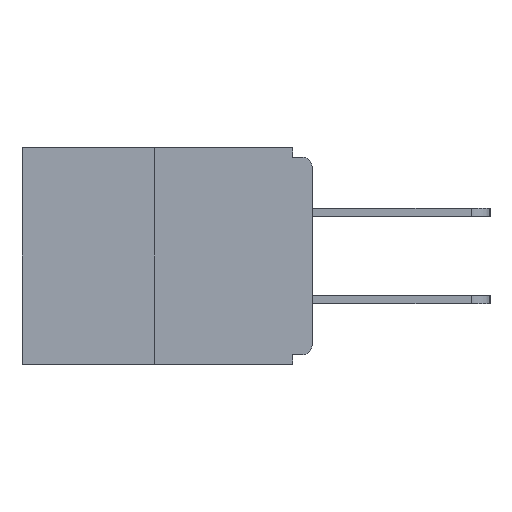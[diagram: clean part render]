
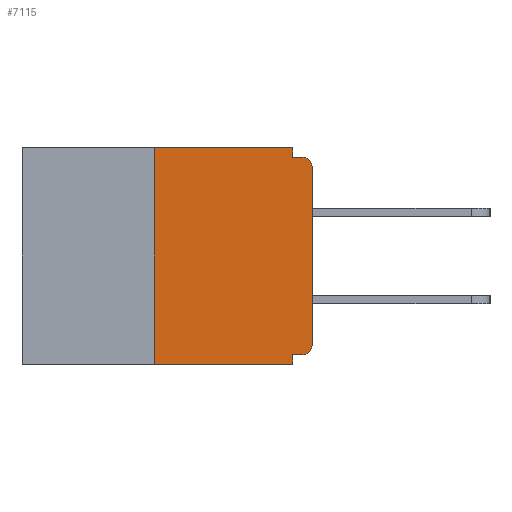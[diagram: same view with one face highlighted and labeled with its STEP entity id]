
A CAD part, left-side view. The second image highlights one B-rep face of the part: STEP entity #7115.
In plain terms, the highlighted planar face has unit normal (-1, 0, 0).
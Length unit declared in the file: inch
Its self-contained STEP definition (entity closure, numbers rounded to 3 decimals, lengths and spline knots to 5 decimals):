
#530 = AXIS2_PLACEMENT_3D ( 'NONE', #10379, #1969, #13027 ) ;
#532 = DIRECTION ( 'NONE',  ( 0., 0., -1. ) ) ;
#1036 = VECTOR ( 'NONE', #11976, 39.37008 ) ;
#1302 = VERTEX_POINT ( 'NONE', #10749 ) ;
#1969 = DIRECTION ( 'NONE',  ( -1., 0., 0. ) ) ;
#2118 = DIRECTION ( 'NONE',  ( 0., 0., -1. ) ) ;
#2387 = VERTEX_POINT ( 'NONE', #3374 ) ;
#2588 = EDGE_CURVE ( 'NONE', #21334, #2387, #24659, .T. ) ;
#2692 = LINE ( 'NONE', #12951, #17182 ) ;
#2912 = VECTOR ( 'NONE', #4541, 39.37008 ) ;
#3039 = ORIENTED_EDGE ( 'NONE', *, *, #25004, .F. ) ;
#3374 = CARTESIAN_POINT ( 'NONE',  ( 0., 0., -0.313 ) ) ;
#3795 = LINE ( 'NONE', #12334, #17183 ) ;
#4541 = DIRECTION ( 'NONE',  ( 0., -1., 0. ) ) ;
#4907 = CARTESIAN_POINT ( 'NONE',  ( 0., 0.46, 0. ) ) ;
#5122 = CARTESIAN_POINT ( 'NONE',  ( 0., 0.25, 0. ) ) ;
#5744 = EDGE_CURVE ( 'NONE', #2387, #20302, #27054, .T. ) ;
#6652 = LINE ( 'NONE', #24101, #2912 ) ;
#6734 = EDGE_LOOP ( 'NONE', ( #27359, #13438, #10868, #3039, #10901, #21600, #6792, #21544, #21994, #18970 ) ) ;
#6792 = ORIENTED_EDGE ( 'NONE', *, *, #5744, .T. ) ;
#7115 = ADVANCED_FACE ( 'NONE', ( #13035 ), #15799, .F. ) ;
#8331 = CARTESIAN_POINT ( 'NONE',  ( 0., 0.015, -0.015 ) ) ;
#9559 = DIRECTION ( 'NONE',  ( 0., 0., -1. ) ) ;
#9563 = EDGE_CURVE ( 'NONE', #1302, #16750, #18788, .T. ) ;
#9677 = EDGE_CURVE ( 'NONE', #20302, #19999, #21326, .T. ) ;
#10379 = CARTESIAN_POINT ( 'NONE',  ( 0., 0.015, -0.313 ) ) ;
#10389 = CARTESIAN_POINT ( 'NONE',  ( 0., 0.015, -0.03 ) ) ;
#10551 = VERTEX_POINT ( 'NONE', #13219 ) ;
#10749 = CARTESIAN_POINT ( 'NONE',  ( 0., 0.25, -0.343 ) ) ;
#10825 = EDGE_CURVE ( 'NONE', #21334, #10551, #20595, .T. ) ;
#10868 = ORIENTED_EDGE ( 'NONE', *, *, #9563, .T. ) ;
#10901 = ORIENTED_EDGE ( 'NONE', *, *, #10825, .F. ) ;
#11485 = EDGE_CURVE ( 'NONE', #17438, #13704, #26472, .T. ) ;
#11976 = DIRECTION ( 'NONE',  ( 0., 0., 1. ) ) ;
#12334 = CARTESIAN_POINT ( 'NONE',  ( 0., 0.031, -0.343 ) ) ;
#12756 = CARTESIAN_POINT ( 'NONE',  ( 0., 0., -0.03 ) ) ;
#12951 = CARTESIAN_POINT ( 'NONE',  ( 0., 0., -0.015 ) ) ;
#13027 = DIRECTION ( 'NONE',  ( 0., 0., -1. ) ) ;
#13035 = FACE_OUTER_BOUND ( 'NONE', #6734, .T. ) ;
#13176 = VECTOR ( 'NONE', #9559, 39.37008 ) ;
#13219 = CARTESIAN_POINT ( 'NONE',  ( 0., 0.031, -0.328 ) ) ;
#13438 = ORIENTED_EDGE ( 'NONE', *, *, #25733, .F. ) ;
#13512 = CARTESIAN_POINT ( 'NONE',  ( 0., 0.031, -0.343 ) ) ;
#13646 = VECTOR ( 'NONE', #22732, 39.37008 ) ;
#13704 = VERTEX_POINT ( 'NONE', #26595 ) ;
#14229 = LINE ( 'NONE', #5122, #13646 ) ;
#14479 = CARTESIAN_POINT ( 'NONE',  ( 0., 0., 0. ) ) ;
#15028 = CARTESIAN_POINT ( 'NONE',  ( 0., 0.25, 0. ) ) ;
#15365 = CARTESIAN_POINT ( 'NONE',  ( 0., 0.031, 0. ) ) ;
#15575 = VECTOR ( 'NONE', #20725, 39.37008 ) ;
#15799 = PLANE ( 'NONE',  #23868 ) ;
#15867 = CARTESIAN_POINT ( 'NONE',  ( 0., 0.031, 0. ) ) ;
#16119 = CARTESIAN_POINT ( 'NONE',  ( 0., 0., -0.328 ) ) ;
#16419 = VECTOR ( 'NONE', #27155, 39.37008 ) ;
#16750 = VERTEX_POINT ( 'NONE', #13512 ) ;
#17182 = VECTOR ( 'NONE', #26037, 39.37008 ) ;
#17183 = VECTOR ( 'NONE', #20855, 39.37008 ) ;
#17438 = VERTEX_POINT ( 'NONE', #15365 ) ;
#18788 = LINE ( 'NONE', #27289, #16419 ) ;
#18970 = ORIENTED_EDGE ( 'NONE', *, *, #11485, .F. ) ;
#19999 = VERTEX_POINT ( 'NONE', #8331 ) ;
#20302 = VERTEX_POINT ( 'NONE', #12756 ) ;
#20595 = LINE ( 'NONE', #16119, #15575 ) ;
#20725 = DIRECTION ( 'NONE',  ( 0., 1., 0. ) ) ;
#20855 = DIRECTION ( 'NONE',  ( 0., 0., -1. ) ) ;
#21326 = CIRCLE ( 'NONE', #23538, 0.015 ) ;
#21334 = VERTEX_POINT ( 'NONE', #26174 ) ;
#21544 = ORIENTED_EDGE ( 'NONE', *, *, #9677, .T. ) ;
#21600 = ORIENTED_EDGE ( 'NONE', *, *, #2588, .T. ) ;
#21994 = ORIENTED_EDGE ( 'NONE', *, *, #23009, .F. ) ;
#22732 = DIRECTION ( 'NONE',  ( 0., 0., 1. ) ) ;
#22814 = VERTEX_POINT ( 'NONE', #15028 ) ;
#23009 = EDGE_CURVE ( 'NONE', #13704, #19999, #2692, .T. ) ;
#23357 = DIRECTION ( 'NONE',  ( -1., 0., 0. ) ) ;
#23538 = AXIS2_PLACEMENT_3D ( 'NONE', #10389, #23357, #2118 ) ;
#23868 = AXIS2_PLACEMENT_3D ( 'NONE', #4907, #24176, #532 ) ;
#24101 = CARTESIAN_POINT ( 'NONE',  ( 0., 0.46, 0. ) ) ;
#24176 = DIRECTION ( 'NONE',  ( 1., 0., 0. ) ) ;
#24659 = CIRCLE ( 'NONE', #530, 0.015 ) ;
#25004 = EDGE_CURVE ( 'NONE', #10551, #16750, #3795, .T. ) ;
#25733 = EDGE_CURVE ( 'NONE', #1302, #22814, #14229, .T. ) ;
#26037 = DIRECTION ( 'NONE',  ( 0., -1., 0. ) ) ;
#26045 = EDGE_CURVE ( 'NONE', #22814, #17438, #6652, .T. ) ;
#26174 = CARTESIAN_POINT ( 'NONE',  ( 0., 0.015, -0.328 ) ) ;
#26472 = LINE ( 'NONE', #15867, #13176 ) ;
#26595 = CARTESIAN_POINT ( 'NONE',  ( 0., 0.031, -0.015 ) ) ;
#27054 = LINE ( 'NONE', #14479, #1036 ) ;
#27155 = DIRECTION ( 'NONE',  ( 0., -1., 0. ) ) ;
#27289 = CARTESIAN_POINT ( 'NONE',  ( 0., 0.46, -0.343 ) ) ;
#27359 = ORIENTED_EDGE ( 'NONE', *, *, #26045, .F. ) ;
